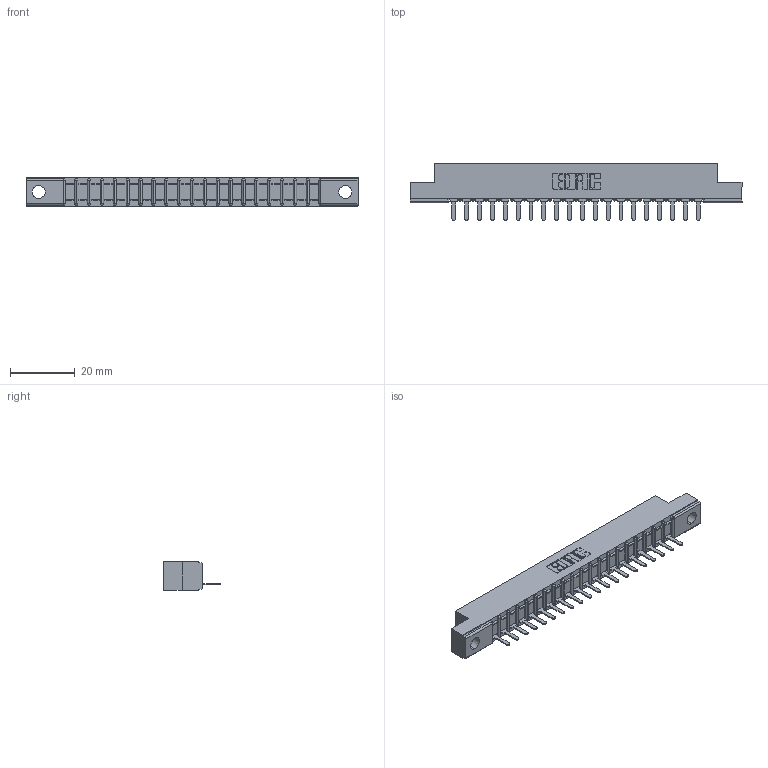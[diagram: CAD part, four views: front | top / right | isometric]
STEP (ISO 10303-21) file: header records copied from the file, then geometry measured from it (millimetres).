
FILE_DESCRIPTION (( 'STEP AP203' ), '1' );
FILE_NAME ('307-020-521-104.STEP', '2019-09-04T23:01:23', ( '' ), ( '' ), 'SwSTEP 2.0', 'SolidWorks 2016', '' );
FILE_SCHEMA (( 'CONFIG_CONTROL_DESIGN' ));
Length unit declared in the file: inch
Products named in the file (3): 307 Part_.156 Dia Mounting Holes; 307-020-521-104; 307-290-002_521
Assembly tree (21 placements, depth 2):
  307-020-521-104
    307 Part_.156 Dia Mounting Holes
    307-290-002_521  x20
Bounding box: 102.26 x 17.42 x 8.71 mm (x, y, z)
Volume: 6645.2 mm3; surface area: 11878.1 mm2
Topology: 21 solids, 21 shells, 1633 faces, 4999 edges, 3274 vertices
Faces by surface type: plane 984, cylinder 607, sphere 42
Entity records: 20994 total; most frequent: CARTESIAN_POINT 3542, ORIENTED_EDGE 3530, DIRECTION 3443, EDGE_CURVE 1765, VECTOR 1349, LINE 1349, VERTEX_POINT 1146, AXIS2_PLACEMENT_3D 1047
